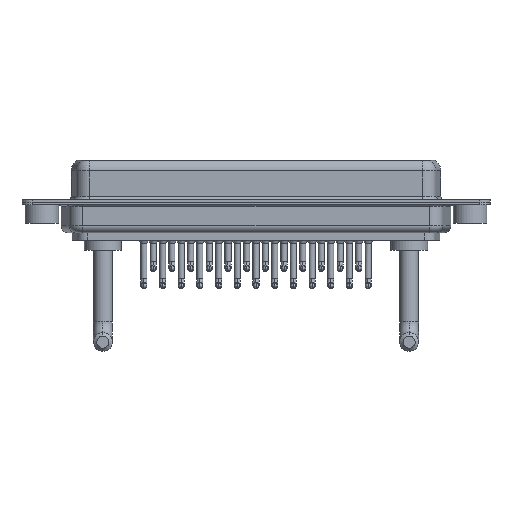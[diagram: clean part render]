
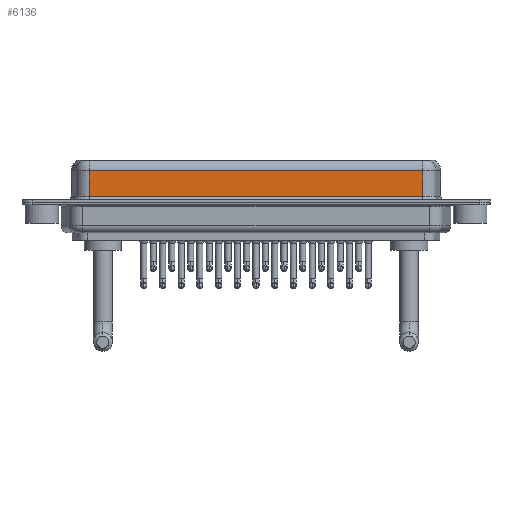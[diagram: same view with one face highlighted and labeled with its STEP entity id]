
A CAD part, front view. The second image highlights one B-rep face of the part: STEP entity #6136.
In plain terms, the highlighted planar face has unit normal (0, -1, 0).
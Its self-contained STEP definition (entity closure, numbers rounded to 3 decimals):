
#316 = VERTEX_POINT ( 'NONE', #17825 ) ;
#2871 = LINE ( 'NONE', #10528, #22301 ) ;
#3974 = ORIENTED_EDGE ( 'NONE', *, *, #12575, .T. ) ;
#4232 = VERTEX_POINT ( 'NONE', #5098 ) ;
#4517 = CARTESIAN_POINT ( 'NONE',  ( 56.462, -3.95, 0.9 ) ) ;
#5098 = CARTESIAN_POINT ( 'NONE',  ( 7.038, -3.95, 4.65 ) ) ;
#6136 = ADVANCED_FACE ( 'NONE', ( #22154 ), #10358, .F. ) ;
#6956 = CARTESIAN_POINT ( 'NONE',  ( 56.462, -3.95, 0.9 ) ) ;
#6982 = AXIS2_PLACEMENT_3D ( 'NONE', #10492, #16012, #11993 ) ;
#7078 = DIRECTION ( 'NONE',  ( -1., 0., 0. ) ) ;
#8713 = LINE ( 'NONE', #24385, #22694 ) ;
#10358 = PLANE ( 'NONE',  #6982 ) ;
#10492 = CARTESIAN_POINT ( 'NONE',  ( 56.462, -3.95, 6.4 ) ) ;
#10528 = CARTESIAN_POINT ( 'NONE',  ( 56.462, -3.95, 6.4 ) ) ;
#10968 = DIRECTION ( 'NONE',  ( 1., 0., 0. ) ) ;
#11516 = EDGE_LOOP ( 'NONE', ( #21617, #17735, #3974, #14437 ) ) ;
#11993 = DIRECTION ( 'NONE',  ( 0., 0., 1. ) ) ;
#12575 = EDGE_CURVE ( 'NONE', #4232, #17632, #18652, .T. ) ;
#12634 = DIRECTION ( 'NONE',  ( 0., 0., -1. ) ) ;
#12924 = EDGE_CURVE ( 'NONE', #316, #4232, #8713, .T. ) ;
#13323 = EDGE_CURVE ( 'NONE', #316, #16386, #2871, .T. ) ;
#14437 = ORIENTED_EDGE ( 'NONE', *, *, #21586, .T. ) ;
#15797 = VECTOR ( 'NONE', #10968, 1000. ) ;
#16012 = DIRECTION ( 'NONE',  ( 0., 1., 0. ) ) ;
#16386 = VERTEX_POINT ( 'NONE', #4517 ) ;
#16500 = LINE ( 'NONE', #6956, #15797 ) ;
#16777 = CARTESIAN_POINT ( 'NONE',  ( 7.038, -3.95, 6.4 ) ) ;
#17632 = VERTEX_POINT ( 'NONE', #19131 ) ;
#17735 = ORIENTED_EDGE ( 'NONE', *, *, #12924, .T. ) ;
#17825 = CARTESIAN_POINT ( 'NONE',  ( 56.462, -3.95, 4.65 ) ) ;
#18652 = LINE ( 'NONE', #16777, #21492 ) ;
#19131 = CARTESIAN_POINT ( 'NONE',  ( 7.038, -3.95, 0.9 ) ) ;
#21492 = VECTOR ( 'NONE', #12634, 1000. ) ;
#21586 = EDGE_CURVE ( 'NONE', #17632, #16386, #16500, .T. ) ;
#21617 = ORIENTED_EDGE ( 'NONE', *, *, #13323, .F. ) ;
#22154 = FACE_OUTER_BOUND ( 'NONE', #11516, .T. ) ;
#22191 = DIRECTION ( 'NONE',  ( 0., 0., -1. ) ) ;
#22301 = VECTOR ( 'NONE', #22191, 1000. ) ;
#22694 = VECTOR ( 'NONE', #7078, 1000. ) ;
#24385 = CARTESIAN_POINT ( 'NONE',  ( 56.462, -3.95, 4.65 ) ) ;
